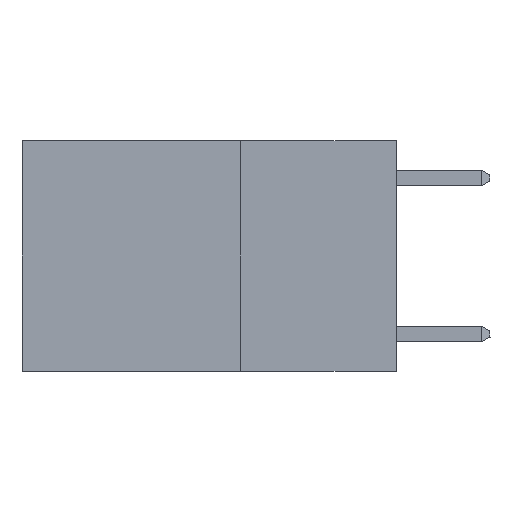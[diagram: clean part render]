
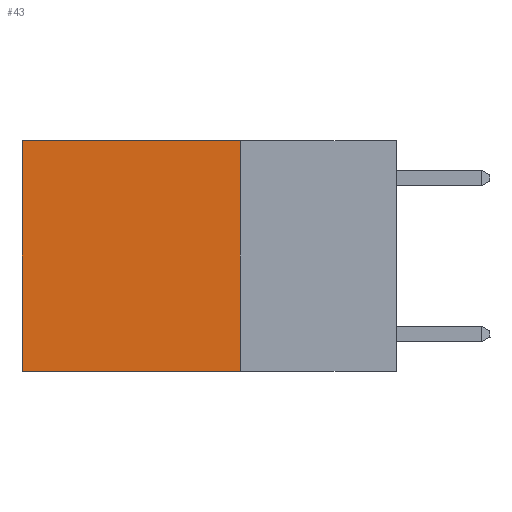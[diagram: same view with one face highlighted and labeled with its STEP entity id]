
A CAD part, left-side view. The second image highlights one B-rep face of the part: STEP entity #43.
In plain terms, the highlighted planar face has unit normal (-1, 0, 0).
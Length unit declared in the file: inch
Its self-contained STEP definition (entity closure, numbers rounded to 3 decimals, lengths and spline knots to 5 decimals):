
#43 = ADVANCED_FACE ( 'NONE', ( #26257 ), #6188, .F. ) ;
#745 = VERTEX_POINT ( 'NONE', #17919 ) ;
#1615 = VERTEX_POINT ( 'NONE', #17459 ) ;
#1983 = DIRECTION ( 'NONE',  ( 0., 0., -1. ) ) ;
#3004 = EDGE_LOOP ( 'NONE', ( #24328, #7945, #4277, #3736 ) ) ;
#3736 = ORIENTED_EDGE ( 'NONE', *, *, #11076, .T. ) ;
#3772 = CARTESIAN_POINT ( 'NONE',  ( 0.2625, 0.25, 0. ) ) ;
#3866 = CARTESIAN_POINT ( 'NONE',  ( 0.2625, 0.25, 0. ) ) ;
#4277 = ORIENTED_EDGE ( 'NONE', *, *, #19938, .F. ) ;
#5100 = VERTEX_POINT ( 'NONE', #21095 ) ;
#6188 = PLANE ( 'NONE',  #13025 ) ;
#7945 = ORIENTED_EDGE ( 'NONE', *, *, #24095, .F. ) ;
#9087 = VECTOR ( 'NONE', #1983, 39.37008 ) ;
#10504 = VECTOR ( 'NONE', #12387, 39.37008 ) ;
#11076 = EDGE_CURVE ( 'NONE', #745, #1615, #19595, .T. ) ;
#12387 = DIRECTION ( 'NONE',  ( 0., 1., 0. ) ) ;
#13025 = AXIS2_PLACEMENT_3D ( 'NONE', #3866, #24711, #14560 ) ;
#13448 = VERTEX_POINT ( 'NONE', #17835 ) ;
#14525 = EDGE_CURVE ( 'NONE', #1615, #5100, #26685, .T. ) ;
#14560 = DIRECTION ( 'NONE',  ( 0., 0., -1. ) ) ;
#14731 = CARTESIAN_POINT ( 'NONE',  ( 0.2625, 0.25, -0.37 ) ) ;
#14742 = LINE ( 'NONE', #3772, #9087 ) ;
#15657 = DIRECTION ( 'NONE',  ( 0., 0., -1. ) ) ;
#16917 = LINE ( 'NONE', #14731, #10504 ) ;
#17459 = CARTESIAN_POINT ( 'NONE',  ( 0.2625, 0.6, 0. ) ) ;
#17835 = CARTESIAN_POINT ( 'NONE',  ( 0.2625, 0.25, -0.37 ) ) ;
#17867 = VECTOR ( 'NONE', #15657, 39.37008 ) ;
#17919 = CARTESIAN_POINT ( 'NONE',  ( 0.2625, 0.25, 0. ) ) ;
#19595 = LINE ( 'NONE', #21258, #20420 ) ;
#19938 = EDGE_CURVE ( 'NONE', #745, #13448, #14742, .T. ) ;
#20420 = VECTOR ( 'NONE', #21780, 39.37008 ) ;
#21095 = CARTESIAN_POINT ( 'NONE',  ( 0.2625, 0.6, -0.37 ) ) ;
#21258 = CARTESIAN_POINT ( 'NONE',  ( 0.2625, 0.25, 0. ) ) ;
#21780 = DIRECTION ( 'NONE',  ( 0., 1., 0. ) ) ;
#24095 = EDGE_CURVE ( 'NONE', #13448, #5100, #16917, .T. ) ;
#24328 = ORIENTED_EDGE ( 'NONE', *, *, #14525, .T. ) ;
#24711 = DIRECTION ( 'NONE',  ( 1., 0., 0. ) ) ;
#25187 = CARTESIAN_POINT ( 'NONE',  ( 0.2625, 0.6, 0. ) ) ;
#26257 = FACE_OUTER_BOUND ( 'NONE', #3004, .T. ) ;
#26685 = LINE ( 'NONE', #25187, #17867 ) ;
